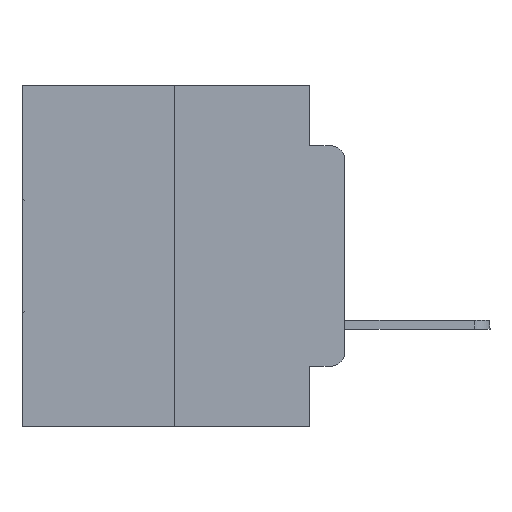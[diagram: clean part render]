
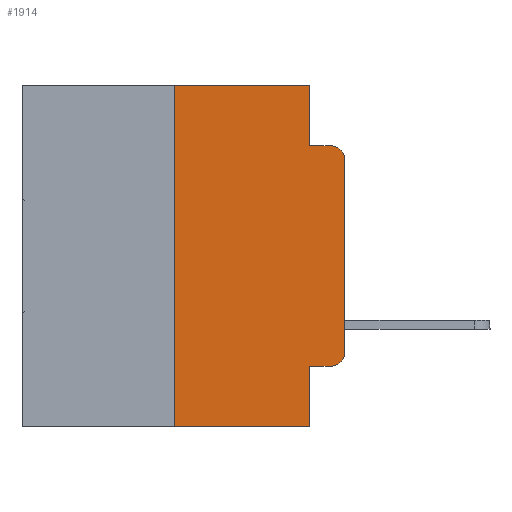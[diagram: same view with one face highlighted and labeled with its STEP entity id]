
A CAD part, left-side view. The second image highlights one B-rep face of the part: STEP entity #1914.
In plain terms, the highlighted planar face has unit normal (-1, 0, 0).
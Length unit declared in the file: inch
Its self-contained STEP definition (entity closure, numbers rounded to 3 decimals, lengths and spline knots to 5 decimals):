
#108 = CARTESIAN_POINT ( 'NONE',  ( 0., 0.051, 0. ) ) ;
#958 = CARTESIAN_POINT ( 'NONE',  ( 0., 0.051, -0.0885 ) ) ;
#1025 = CARTESIAN_POINT ( 'NONE',  ( 0., 0.051, -0.4115 ) ) ;
#1061 = FACE_OUTER_BOUND ( 'NONE', #9164, .T. ) ;
#1201 = PLANE ( 'NONE',  #17949 ) ;
#1311 = VERTEX_POINT ( 'NONE', #6206 ) ;
#1355 = DIRECTION ( 'NONE',  ( 0., 0., -1. ) ) ;
#1914 = ADVANCED_FACE ( 'NONE', ( #1061 ), #1201, .F. ) ;
#2174 = CARTESIAN_POINT ( 'NONE',  ( 0., 0.051, -0.4115 ) ) ;
#2183 = VERTEX_POINT ( 'NONE', #14033 ) ;
#2684 = ORIENTED_EDGE ( 'NONE', *, *, #11337, .T. ) ;
#2875 = EDGE_CURVE ( 'NONE', #23953, #1311, #28028, .T. ) ;
#3151 = ORIENTED_EDGE ( 'NONE', *, *, #2875, .F. ) ;
#3284 = DIRECTION ( 'NONE',  ( 0., -1., 0. ) ) ;
#3529 = CARTESIAN_POINT ( 'NONE',  ( 0., 0.051, 0. ) ) ;
#3583 = VECTOR ( 'NONE', #21171, 39.37008 ) ;
#3669 = DIRECTION ( 'NONE',  ( 0., -1., 0. ) ) ;
#4700 = EDGE_CURVE ( 'NONE', #19459, #2183, #6584, .T. ) ;
#5499 = LINE ( 'NONE', #23162, #18633 ) ;
#5536 = EDGE_CURVE ( 'NONE', #18187, #19459, #16968, .T. ) ;
#5769 = EDGE_CURVE ( 'NONE', #15560, #25111, #7837, .T. ) ;
#5863 = ORIENTED_EDGE ( 'NONE', *, *, #4700, .T. ) ;
#6001 = LINE ( 'NONE', #3529, #16236 ) ;
#6192 = DIRECTION ( 'NONE',  ( 0., -1., 0. ) ) ;
#6206 = CARTESIAN_POINT ( 'NONE',  ( 0., 0.051, -0.0885 ) ) ;
#6531 = VERTEX_POINT ( 'NONE', #23693 ) ;
#6564 = CARTESIAN_POINT ( 'NONE',  ( 0., 0.02, -0.0885 ) ) ;
#6584 = CIRCLE ( 'NONE', #10251, 0.02 ) ;
#7128 = CARTESIAN_POINT ( 'NONE',  ( 0., 0.051, -0.5 ) ) ;
#7394 = CARTESIAN_POINT ( 'NONE',  ( 0., 0.02, -0.1085 ) ) ;
#7792 = ORIENTED_EDGE ( 'NONE', *, *, #10885, .F. ) ;
#7837 = CIRCLE ( 'NONE', #27711, 0.02 ) ;
#8396 = CARTESIAN_POINT ( 'NONE',  ( 0., 0.25, 0. ) ) ;
#9164 = EDGE_LOOP ( 'NONE', ( #2684, #11815, #7792, #3151, #10683, #17485, #24457, #24555, #10281, #5863 ) ) ;
#9892 = DIRECTION ( 'NONE',  ( 0., 0., -1. ) ) ;
#10119 = DIRECTION ( 'NONE',  ( 0., 0., -1. ) ) ;
#10251 = AXIS2_PLACEMENT_3D ( 'NONE', #16648, #27921, #10119 ) ;
#10281 = ORIENTED_EDGE ( 'NONE', *, *, #5536, .T. ) ;
#10683 = ORIENTED_EDGE ( 'NONE', *, *, #14845, .F. ) ;
#10885 = EDGE_CURVE ( 'NONE', #1311, #25111, #25145, .T. ) ;
#11337 = EDGE_CURVE ( 'NONE', #2183, #15560, #17695, .T. ) ;
#11648 = VECTOR ( 'NONE', #3284, 39.37008 ) ;
#11815 = ORIENTED_EDGE ( 'NONE', *, *, #5769, .T. ) ;
#11866 = DIRECTION ( 'NONE',  ( -1., 0., 0. ) ) ;
#12356 = DIRECTION ( 'NONE',  ( 1., 0., 0. ) ) ;
#12466 = VECTOR ( 'NONE', #3669, 39.37008 ) ;
#13332 = CARTESIAN_POINT ( 'NONE',  ( 0., 0.02, -0.4115 ) ) ;
#14033 = CARTESIAN_POINT ( 'NONE',  ( 0., 0., -0.3915 ) ) ;
#14136 = DIRECTION ( 'NONE',  ( 0., 0., -1. ) ) ;
#14234 = CARTESIAN_POINT ( 'NONE',  ( 0., 0.473, 0. ) ) ;
#14604 = DIRECTION ( 'NONE',  ( 0., 0., 1. ) ) ;
#14730 = LINE ( 'NONE', #15013, #23412 ) ;
#14845 = EDGE_CURVE ( 'NONE', #20905, #23953, #22922, .T. ) ;
#14927 = CARTESIAN_POINT ( 'NONE',  ( 0., 0., 0. ) ) ;
#15013 = CARTESIAN_POINT ( 'NONE',  ( 0., 0.473, -0.5 ) ) ;
#15560 = VERTEX_POINT ( 'NONE', #26298 ) ;
#15885 = EDGE_CURVE ( 'NONE', #18187, #19237, #6001, .T. ) ;
#16236 = VECTOR ( 'NONE', #1355, 39.37008 ) ;
#16648 = CARTESIAN_POINT ( 'NONE',  ( 0., 0.02, -0.3915 ) ) ;
#16968 = LINE ( 'NONE', #1025, #3583 ) ;
#17485 = ORIENTED_EDGE ( 'NONE', *, *, #18044, .F. ) ;
#17695 = LINE ( 'NONE', #14927, #23477 ) ;
#17949 = AXIS2_PLACEMENT_3D ( 'NONE', #22926, #12356, #9892 ) ;
#18044 = EDGE_CURVE ( 'NONE', #6531, #20905, #5499, .T. ) ;
#18187 = VERTEX_POINT ( 'NONE', #2174 ) ;
#18633 = VECTOR ( 'NONE', #14604, 39.37008 ) ;
#19237 = VERTEX_POINT ( 'NONE', #7128 ) ;
#19459 = VERTEX_POINT ( 'NONE', #13332 ) ;
#20905 = VERTEX_POINT ( 'NONE', #8396 ) ;
#21171 = DIRECTION ( 'NONE',  ( 0., -1., 0. ) ) ;
#22316 = DIRECTION ( 'NONE',  ( 0., 0., -1. ) ) ;
#22922 = LINE ( 'NONE', #14234, #12466 ) ;
#22926 = CARTESIAN_POINT ( 'NONE',  ( 0., 0.473, 0. ) ) ;
#23118 = CARTESIAN_POINT ( 'NONE',  ( 0., 0.051, 0. ) ) ;
#23162 = CARTESIAN_POINT ( 'NONE',  ( 0., 0.25, 0. ) ) ;
#23412 = VECTOR ( 'NONE', #6192, 39.37008 ) ;
#23477 = VECTOR ( 'NONE', #25942, 39.37008 ) ;
#23693 = CARTESIAN_POINT ( 'NONE',  ( 0., 0.25, -0.5 ) ) ;
#23953 = VERTEX_POINT ( 'NONE', #108 ) ;
#24457 = ORIENTED_EDGE ( 'NONE', *, *, #27029, .T. ) ;
#24555 = ORIENTED_EDGE ( 'NONE', *, *, #15885, .F. ) ;
#25111 = VERTEX_POINT ( 'NONE', #6564 ) ;
#25145 = LINE ( 'NONE', #958, #11648 ) ;
#25383 = VECTOR ( 'NONE', #14136, 39.37008 ) ;
#25942 = DIRECTION ( 'NONE',  ( 0., 0., 1. ) ) ;
#26298 = CARTESIAN_POINT ( 'NONE',  ( 0., 0., -0.1085 ) ) ;
#27029 = EDGE_CURVE ( 'NONE', #6531, #19237, #14730, .T. ) ;
#27711 = AXIS2_PLACEMENT_3D ( 'NONE', #7394, #11866, #22316 ) ;
#27921 = DIRECTION ( 'NONE',  ( -1., 0., 0. ) ) ;
#28028 = LINE ( 'NONE', #23118, #25383 ) ;
